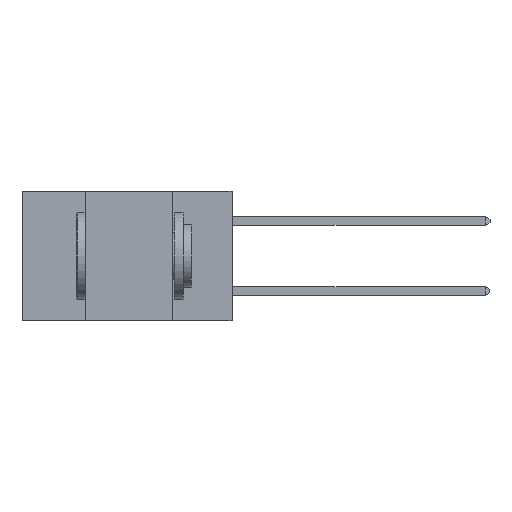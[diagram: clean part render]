
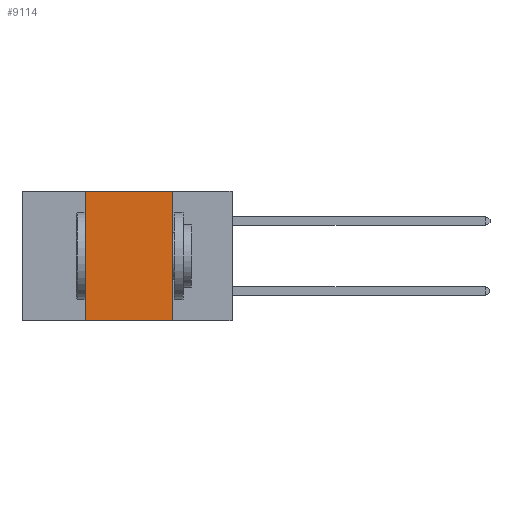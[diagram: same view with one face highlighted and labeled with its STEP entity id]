
A CAD part, left-side view. The second image highlights one B-rep face of the part: STEP entity #9114.
In plain terms, the highlighted planar face has unit normal (-1, 0, 0).
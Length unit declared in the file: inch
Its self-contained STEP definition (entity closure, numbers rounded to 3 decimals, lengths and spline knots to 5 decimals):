
#169 = VERTEX_POINT ( 'NONE', #9487 ) ;
#1649 = ORIENTED_EDGE ( 'NONE', *, *, #15220, .T. ) ;
#2065 = VECTOR ( 'NONE', #8880, 39.37008 ) ;
#2976 = VECTOR ( 'NONE', #18370, 39.37008 ) ;
#3678 = ORIENTED_EDGE ( 'NONE', *, *, #20662, .F. ) ;
#5118 = VERTEX_POINT ( 'NONE', #14195 ) ;
#6254 = DIRECTION ( 'NONE',  ( 0., 0., 1. ) ) ;
#6456 = LINE ( 'NONE', #6566, #2976 ) ;
#6471 = EDGE_LOOP ( 'NONE', ( #11559, #3678, #9491, #1649 ) ) ;
#6566 = CARTESIAN_POINT ( 'NONE',  ( 0., 0.17, 0. ) ) ;
#6622 = VERTEX_POINT ( 'NONE', #11713 ) ;
#6629 = LINE ( 'NONE', #12192, #2065 ) ;
#8258 = VERTEX_POINT ( 'NONE', #19349 ) ;
#8880 = DIRECTION ( 'NONE',  ( 0., -1., 0. ) ) ;
#9114 = ADVANCED_FACE ( 'NONE', ( #20587 ), #18182, .F. ) ;
#9415 = EDGE_CURVE ( 'NONE', #5118, #169, #6456, .T. ) ;
#9487 = CARTESIAN_POINT ( 'NONE',  ( 0., 0.17, -0.37 ) ) ;
#9491 = ORIENTED_EDGE ( 'NONE', *, *, #16809, .F. ) ;
#9730 = AXIS2_PLACEMENT_3D ( 'NONE', #19802, #21437, #11476 ) ;
#10249 = VECTOR ( 'NONE', #17120, 39.37008 ) ;
#11476 = DIRECTION ( 'NONE',  ( 0., 0., -1. ) ) ;
#11559 = ORIENTED_EDGE ( 'NONE', *, *, #9415, .F. ) ;
#11713 = CARTESIAN_POINT ( 'NONE',  ( 0., 0.42, 0. ) ) ;
#12192 = CARTESIAN_POINT ( 'NONE',  ( 0., 0.6, 0. ) ) ;
#12272 = LINE ( 'NONE', #12960, #20589 ) ;
#12960 = CARTESIAN_POINT ( 'NONE',  ( 0., 0.42, 0. ) ) ;
#14195 = CARTESIAN_POINT ( 'NONE',  ( 0., 0.17, 0. ) ) ;
#14707 = LINE ( 'NONE', #15372, #10249 ) ;
#15220 = EDGE_CURVE ( 'NONE', #8258, #169, #14707, .T. ) ;
#15372 = CARTESIAN_POINT ( 'NONE',  ( 0., 0.6, -0.37 ) ) ;
#16809 = EDGE_CURVE ( 'NONE', #8258, #6622, #12272, .T. ) ;
#17120 = DIRECTION ( 'NONE',  ( 0., -1., 0. ) ) ;
#18182 = PLANE ( 'NONE',  #9730 ) ;
#18370 = DIRECTION ( 'NONE',  ( 0., 0., -1. ) ) ;
#19349 = CARTESIAN_POINT ( 'NONE',  ( 0., 0.42, -0.37 ) ) ;
#19802 = CARTESIAN_POINT ( 'NONE',  ( 0., 0.6, 0. ) ) ;
#20587 = FACE_OUTER_BOUND ( 'NONE', #6471, .T. ) ;
#20589 = VECTOR ( 'NONE', #6254, 39.37008 ) ;
#20662 = EDGE_CURVE ( 'NONE', #6622, #5118, #6629, .T. ) ;
#21437 = DIRECTION ( 'NONE',  ( 1., 0., 0. ) ) ;
